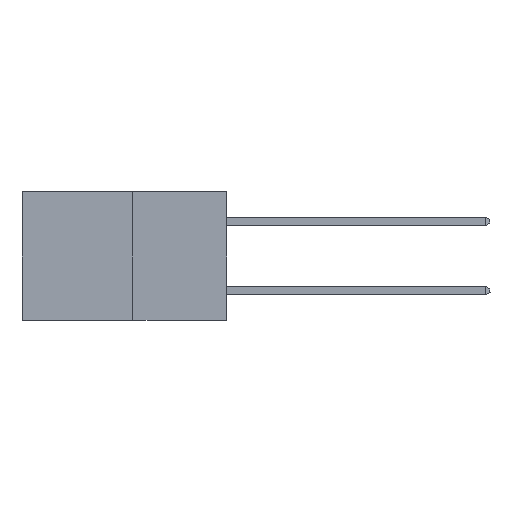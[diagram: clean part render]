
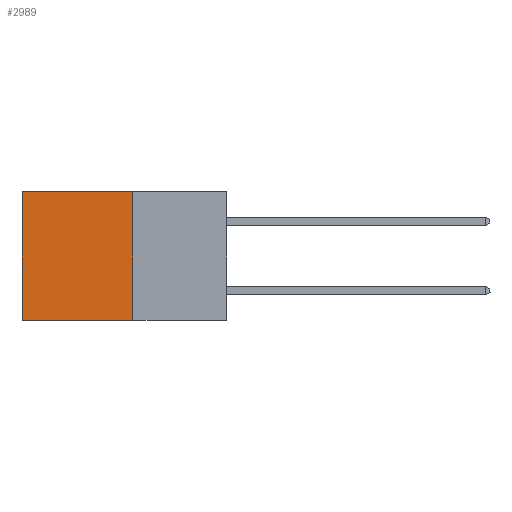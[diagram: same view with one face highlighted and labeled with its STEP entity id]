
A CAD part, left-side view. The second image highlights one B-rep face of the part: STEP entity #2989.
In plain terms, the highlighted planar face has unit normal (-1, 0, 0).
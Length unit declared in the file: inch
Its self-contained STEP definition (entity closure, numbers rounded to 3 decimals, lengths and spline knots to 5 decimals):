
#843 = CARTESIAN_POINT ( 'NONE',  ( 0.277, 0.27, 0. ) ) ;
#1709 = EDGE_LOOP ( 'NONE', ( #4217, #11248, #19447, #14324 ) ) ;
#1837 = CARTESIAN_POINT ( 'NONE',  ( 0.277, 0.59, -0.37 ) ) ;
#2021 = CARTESIAN_POINT ( 'NONE',  ( 0.277, 0.27, -0.37 ) ) ;
#2989 = ADVANCED_FACE ( 'NONE', ( #21286 ), #18427, .F. ) ;
#4161 = DIRECTION ( 'NONE',  ( 0., 1., 0. ) ) ;
#4172 = VECTOR ( 'NONE', #5884, 39.37008 ) ;
#4217 = ORIENTED_EDGE ( 'NONE', *, *, #7300, .T. ) ;
#4494 = CARTESIAN_POINT ( 'NONE',  ( 0.277, 0.27, 0. ) ) ;
#4611 = EDGE_CURVE ( 'NONE', #17466, #13228, #18498, .T. ) ;
#5884 = DIRECTION ( 'NONE',  ( 0., 1., 0. ) ) ;
#6132 = CARTESIAN_POINT ( 'NONE',  ( 0.277, 0.27, -0.37 ) ) ;
#6163 = AXIS2_PLACEMENT_3D ( 'NONE', #18527, #15395, #15052 ) ;
#7300 = EDGE_CURVE ( 'NONE', #13228, #7436, #25463, .T. ) ;
#7436 = VERTEX_POINT ( 'NONE', #1837 ) ;
#8205 = DIRECTION ( 'NONE',  ( 0., 0., -1. ) ) ;
#10547 = VERTEX_POINT ( 'NONE', #2021 ) ;
#11248 = ORIENTED_EDGE ( 'NONE', *, *, #13639, .F. ) ;
#11784 = LINE ( 'NONE', #6132, #16035 ) ;
#12928 = VECTOR ( 'NONE', #4161, 39.37008 ) ;
#13228 = VERTEX_POINT ( 'NONE', #17209 ) ;
#13639 = EDGE_CURVE ( 'NONE', #10547, #7436, #15093, .T. ) ;
#14324 = ORIENTED_EDGE ( 'NONE', *, *, #4611, .T. ) ;
#15052 = DIRECTION ( 'NONE',  ( 0., 0., -1. ) ) ;
#15093 = LINE ( 'NONE', #22438, #4172 ) ;
#15395 = DIRECTION ( 'NONE',  ( 1., 0., 0. ) ) ;
#16035 = VECTOR ( 'NONE', #8205, 39.37008 ) ;
#17209 = CARTESIAN_POINT ( 'NONE',  ( 0.277, 0.59, 0. ) ) ;
#17466 = VERTEX_POINT ( 'NONE', #843 ) ;
#18427 = PLANE ( 'NONE',  #6163 ) ;
#18498 = LINE ( 'NONE', #4494, #12928 ) ;
#18527 = CARTESIAN_POINT ( 'NONE',  ( 0.277, 0.27, -0.37 ) ) ;
#19390 = VECTOR ( 'NONE', #19944, 39.37008 ) ;
#19447 = ORIENTED_EDGE ( 'NONE', *, *, #21144, .F. ) ;
#19944 = DIRECTION ( 'NONE',  ( 0., 0., -1. ) ) ;
#21144 = EDGE_CURVE ( 'NONE', #17466, #10547, #11784, .T. ) ;
#21286 = FACE_OUTER_BOUND ( 'NONE', #1709, .T. ) ;
#22024 = CARTESIAN_POINT ( 'NONE',  ( 0.277, 0.59, -0.37 ) ) ;
#22438 = CARTESIAN_POINT ( 'NONE',  ( 0.277, 0.27, -0.37 ) ) ;
#25463 = LINE ( 'NONE', #22024, #19390 ) ;
